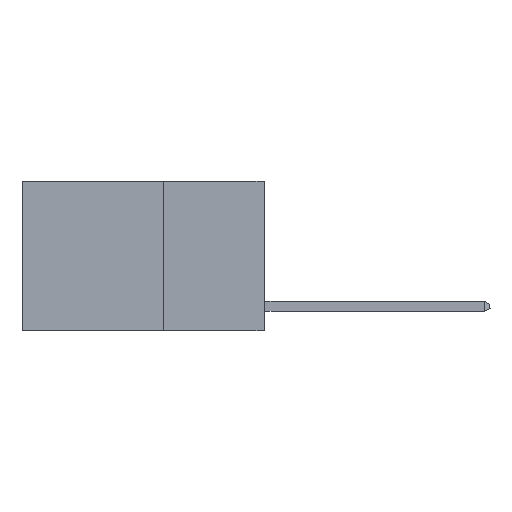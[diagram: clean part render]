
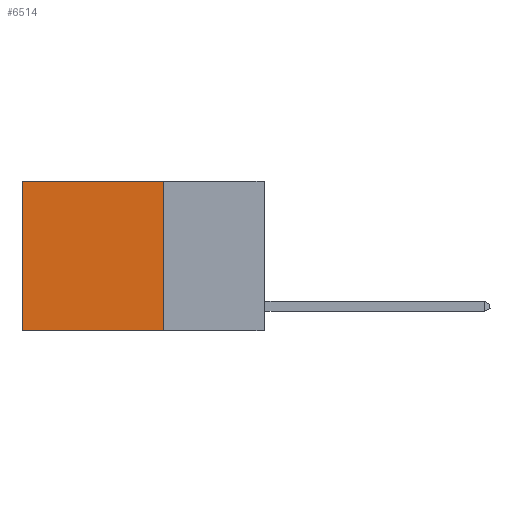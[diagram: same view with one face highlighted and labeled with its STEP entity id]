
A CAD part, left-side view. The second image highlights one B-rep face of the part: STEP entity #6514.
In plain terms, the highlighted planar face has unit normal (-1, 0, 0).
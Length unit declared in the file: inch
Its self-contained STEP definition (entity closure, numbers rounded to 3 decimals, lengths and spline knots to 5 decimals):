
#335 = CARTESIAN_POINT ( 'NONE',  ( 0.2625, 0.6, -0.37 ) ) ;
#1271 = ORIENTED_EDGE ( 'NONE', *, *, #16644, .T. ) ;
#1929 = VECTOR ( 'NONE', #4236, 39.37008 ) ;
#2466 = LINE ( 'NONE', #7622, #2918 ) ;
#2918 = VECTOR ( 'NONE', #9060, 39.37008 ) ;
#3054 = PLANE ( 'NONE',  #4768 ) ;
#3265 = CARTESIAN_POINT ( 'NONE',  ( 0.2625, 0.25, 0. ) ) ;
#3433 = ORIENTED_EDGE ( 'NONE', *, *, #5210, .T. ) ;
#3658 = VERTEX_POINT ( 'NONE', #335 ) ;
#4236 = DIRECTION ( 'NONE',  ( 0., 1., 0. ) ) ;
#4348 = ORIENTED_EDGE ( 'NONE', *, *, #17225, .F. ) ;
#4349 = FACE_OUTER_BOUND ( 'NONE', #11327, .T. ) ;
#4683 = DIRECTION ( 'NONE',  ( 0., 0., -1. ) ) ;
#4768 = AXIS2_PLACEMENT_3D ( 'NONE', #12984, #14421, #5901 ) ;
#4824 = EDGE_CURVE ( 'NONE', #17853, #3658, #18117, .T. ) ;
#5210 = EDGE_CURVE ( 'NONE', #9952, #13034, #12851, .T. ) ;
#5901 = DIRECTION ( 'NONE',  ( 0., 0., -1. ) ) ;
#6432 = VECTOR ( 'NONE', #4683, 39.37008 ) ;
#6508 = CARTESIAN_POINT ( 'NONE',  ( 0.2625, 0.25, -0.37 ) ) ;
#6514 = ADVANCED_FACE ( 'NONE', ( #4349 ), #3054, .F. ) ;
#6860 = VECTOR ( 'NONE', #13662, 39.37008 ) ;
#7365 = CARTESIAN_POINT ( 'NONE',  ( 0.2625, 0.6, 0. ) ) ;
#7622 = CARTESIAN_POINT ( 'NONE',  ( 0.2625, 0.6, 0. ) ) ;
#9060 = DIRECTION ( 'NONE',  ( 0., 0., -1. ) ) ;
#9543 = ORIENTED_EDGE ( 'NONE', *, *, #4824, .F. ) ;
#9952 = VERTEX_POINT ( 'NONE', #16258 ) ;
#10017 = CARTESIAN_POINT ( 'NONE',  ( 0.2625, 0.25, 0. ) ) ;
#11327 = EDGE_LOOP ( 'NONE', ( #1271, #9543, #4348, #3433 ) ) ;
#12851 = LINE ( 'NONE', #10017, #1929 ) ;
#12984 = CARTESIAN_POINT ( 'NONE',  ( 0.2625, 0.25, 0. ) ) ;
#13034 = VERTEX_POINT ( 'NONE', #7365 ) ;
#13057 = CARTESIAN_POINT ( 'NONE',  ( 0.2625, 0.25, -0.37 ) ) ;
#13662 = DIRECTION ( 'NONE',  ( 0., 1., 0. ) ) ;
#14421 = DIRECTION ( 'NONE',  ( 1., 0., 0. ) ) ;
#14878 = LINE ( 'NONE', #3265, #6432 ) ;
#16258 = CARTESIAN_POINT ( 'NONE',  ( 0.2625, 0.25, 0. ) ) ;
#16644 = EDGE_CURVE ( 'NONE', #13034, #3658, #2466, .T. ) ;
#17225 = EDGE_CURVE ( 'NONE', #9952, #17853, #14878, .T. ) ;
#17853 = VERTEX_POINT ( 'NONE', #13057 ) ;
#18117 = LINE ( 'NONE', #6508, #6860 ) ;
